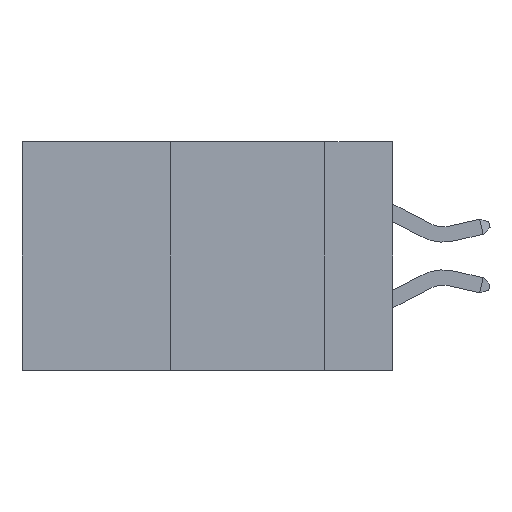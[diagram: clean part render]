
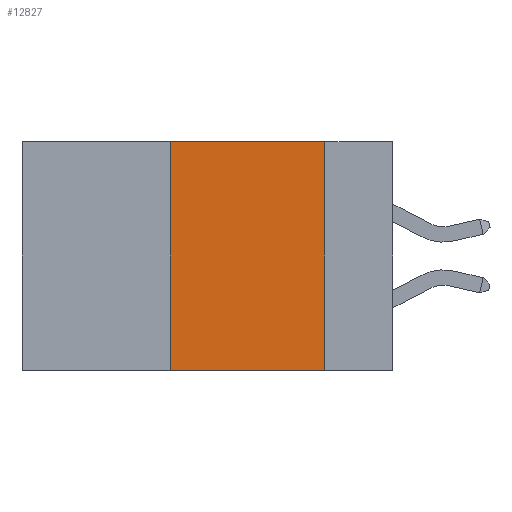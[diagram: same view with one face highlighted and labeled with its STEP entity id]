
A CAD part, left-side view. The second image highlights one B-rep face of the part: STEP entity #12827.
In plain terms, the highlighted planar face has unit normal (-1, 0, 0).
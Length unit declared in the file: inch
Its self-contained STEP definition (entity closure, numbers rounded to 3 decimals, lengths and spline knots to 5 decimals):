
#8 = VERTEX_POINT ( 'NONE', #20881 ) ;
#557 = CARTESIAN_POINT ( 'NONE',  ( 0., 0.36, 0. ) ) ;
#983 = CARTESIAN_POINT ( 'NONE',  ( 0., 0.6, 0. ) ) ;
#2327 = LINE ( 'NONE', #557, #2431 ) ;
#2431 = VECTOR ( 'NONE', #18975, 39.37008 ) ;
#3150 = FACE_OUTER_BOUND ( 'NONE', #25662, .T. ) ;
#5137 = PLANE ( 'NONE',  #11151 ) ;
#5828 = EDGE_CURVE ( 'NONE', #9087, #24803, #25452, .T. ) ;
#6480 = ORIENTED_EDGE ( 'NONE', *, *, #13783, .F. ) ;
#6973 = LINE ( 'NONE', #8989, #13049 ) ;
#7308 = DIRECTION ( 'NONE',  ( 1., 0., 0. ) ) ;
#8349 = VECTOR ( 'NONE', #20168, 39.37008 ) ;
#8989 = CARTESIAN_POINT ( 'NONE',  ( 0., 0.6, 0. ) ) ;
#9087 = VERTEX_POINT ( 'NONE', #22562 ) ;
#9570 = CARTESIAN_POINT ( 'NONE',  ( 0., 0.11, 0. ) ) ;
#10500 = ORIENTED_EDGE ( 'NONE', *, *, #5828, .T. ) ;
#11151 = AXIS2_PLACEMENT_3D ( 'NONE', #983, #7308, #19529 ) ;
#12064 = ORIENTED_EDGE ( 'NONE', *, *, #18729, .F. ) ;
#12827 = ADVANCED_FACE ( 'NONE', ( #3150 ), #5137, .F. ) ;
#13049 = VECTOR ( 'NONE', #17164, 39.37008 ) ;
#13783 = EDGE_CURVE ( 'NONE', #24060, #24803, #14003, .T. ) ;
#14003 = LINE ( 'NONE', #9570, #8349 ) ;
#15716 = DIRECTION ( 'NONE',  ( 0., -1., 0. ) ) ;
#17164 = DIRECTION ( 'NONE',  ( 0., -1., 0. ) ) ;
#17602 = CARTESIAN_POINT ( 'NONE',  ( 0., 0.6, -0.37 ) ) ;
#17621 = CARTESIAN_POINT ( 'NONE',  ( 0., 0.11, 0. ) ) ;
#18729 = EDGE_CURVE ( 'NONE', #8, #24060, #6973, .T. ) ;
#18975 = DIRECTION ( 'NONE',  ( 0., 0., 1. ) ) ;
#19313 = CARTESIAN_POINT ( 'NONE',  ( 0., 0.11, -0.37 ) ) ;
#19407 = ORIENTED_EDGE ( 'NONE', *, *, #21195, .F. ) ;
#19529 = DIRECTION ( 'NONE',  ( 0., 0., -1. ) ) ;
#19836 = VECTOR ( 'NONE', #15716, 39.37008 ) ;
#20168 = DIRECTION ( 'NONE',  ( 0., 0., -1. ) ) ;
#20881 = CARTESIAN_POINT ( 'NONE',  ( 0., 0.36, 0. ) ) ;
#21195 = EDGE_CURVE ( 'NONE', #9087, #8, #2327, .T. ) ;
#22562 = CARTESIAN_POINT ( 'NONE',  ( 0., 0.36, -0.37 ) ) ;
#24060 = VERTEX_POINT ( 'NONE', #17621 ) ;
#24803 = VERTEX_POINT ( 'NONE', #19313 ) ;
#25452 = LINE ( 'NONE', #17602, #19836 ) ;
#25662 = EDGE_LOOP ( 'NONE', ( #6480, #12064, #19407, #10500 ) ) ;
